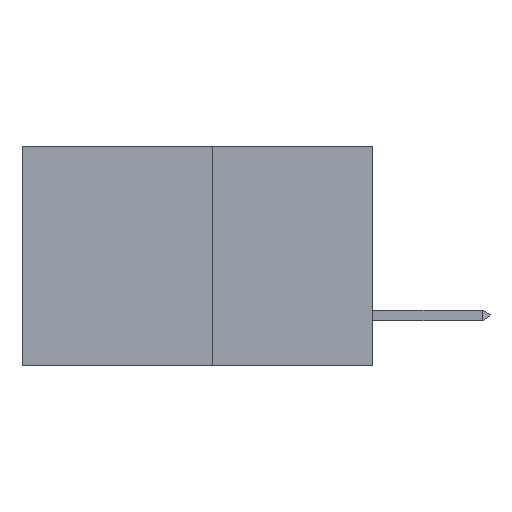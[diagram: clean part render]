
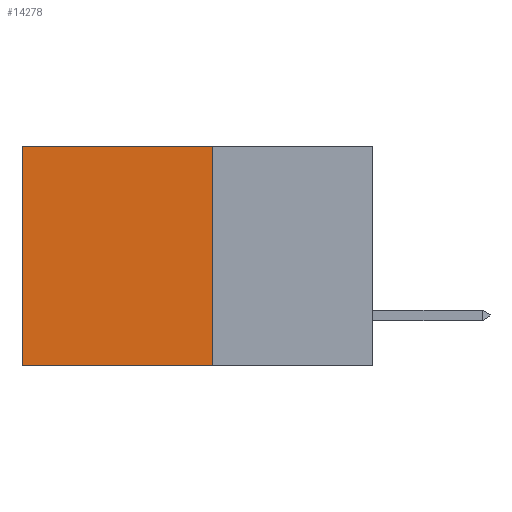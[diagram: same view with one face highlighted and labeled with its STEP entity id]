
A CAD part, left-side view. The second image highlights one B-rep face of the part: STEP entity #14278.
In plain terms, the highlighted planar face has unit normal (-1, 0, 0).
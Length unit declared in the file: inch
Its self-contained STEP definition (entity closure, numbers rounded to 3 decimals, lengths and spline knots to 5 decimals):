
#342 = ORIENTED_EDGE ( 'NONE', *, *, #14026, .F. ) ;
#518 = EDGE_CURVE ( 'NONE', #7030, #1670, #5116, .T. ) ;
#786 = CARTESIAN_POINT ( 'NONE',  ( 0.277, 0.59, -0.37 ) ) ;
#931 = ORIENTED_EDGE ( 'NONE', *, *, #7971, .T. ) ;
#1202 = FACE_OUTER_BOUND ( 'NONE', #6365, .T. ) ;
#1516 = CARTESIAN_POINT ( 'NONE',  ( 0.277, 0.27, -0.37 ) ) ;
#1670 = VERTEX_POINT ( 'NONE', #7050 ) ;
#3522 = CARTESIAN_POINT ( 'NONE',  ( 0.277, 0.59, 0. ) ) ;
#4416 = ORIENTED_EDGE ( 'NONE', *, *, #518, .F. ) ;
#4420 = DIRECTION ( 'NONE',  ( 0., 1., 0. ) ) ;
#4527 = DIRECTION ( 'NONE',  ( 0., 0., -1. ) ) ;
#5116 = LINE ( 'NONE', #1516, #13660 ) ;
#6236 = VERTEX_POINT ( 'NONE', #7730 ) ;
#6365 = EDGE_LOOP ( 'NONE', ( #931, #4416, #342, #6558 ) ) ;
#6558 = ORIENTED_EDGE ( 'NONE', *, *, #7881, .T. ) ;
#7030 = VERTEX_POINT ( 'NONE', #8870 ) ;
#7050 = CARTESIAN_POINT ( 'NONE',  ( 0.277, 0.59, -0.37 ) ) ;
#7730 = CARTESIAN_POINT ( 'NONE',  ( 0.277, 0.27, 0. ) ) ;
#7858 = DIRECTION ( 'NONE',  ( 0., 0., -1. ) ) ;
#7881 = EDGE_CURVE ( 'NONE', #6236, #8256, #10096, .T. ) ;
#7971 = EDGE_CURVE ( 'NONE', #8256, #1670, #8183, .T. ) ;
#8183 = LINE ( 'NONE', #786, #11044 ) ;
#8256 = VERTEX_POINT ( 'NONE', #3522 ) ;
#8870 = CARTESIAN_POINT ( 'NONE',  ( 0.277, 0.27, -0.37 ) ) ;
#8989 = CARTESIAN_POINT ( 'NONE',  ( 0.277, 0.27, -0.37 ) ) ;
#9267 = CARTESIAN_POINT ( 'NONE',  ( 0.277, 0.27, 0. ) ) ;
#10096 = LINE ( 'NONE', #9267, #12181 ) ;
#10206 = DIRECTION ( 'NONE',  ( 0., 0., -1. ) ) ;
#11044 = VECTOR ( 'NONE', #4527, 39.37008 ) ;
#11190 = VECTOR ( 'NONE', #10206, 39.37008 ) ;
#11950 = LINE ( 'NONE', #8989, #11190 ) ;
#12181 = VECTOR ( 'NONE', #4420, 39.37008 ) ;
#12709 = PLANE ( 'NONE',  #13874 ) ;
#13660 = VECTOR ( 'NONE', #14597, 39.37008 ) ;
#13874 = AXIS2_PLACEMENT_3D ( 'NONE', #13909, #15093, #7858 ) ;
#13909 = CARTESIAN_POINT ( 'NONE',  ( 0.277, 0.27, -0.37 ) ) ;
#14026 = EDGE_CURVE ( 'NONE', #6236, #7030, #11950, .T. ) ;
#14278 = ADVANCED_FACE ( 'NONE', ( #1202 ), #12709, .F. ) ;
#14597 = DIRECTION ( 'NONE',  ( 0., 1., 0. ) ) ;
#15093 = DIRECTION ( 'NONE',  ( 1., 0., 0. ) ) ;
